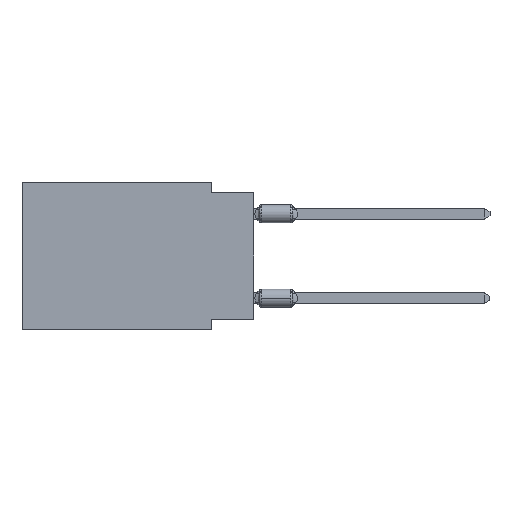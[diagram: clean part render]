
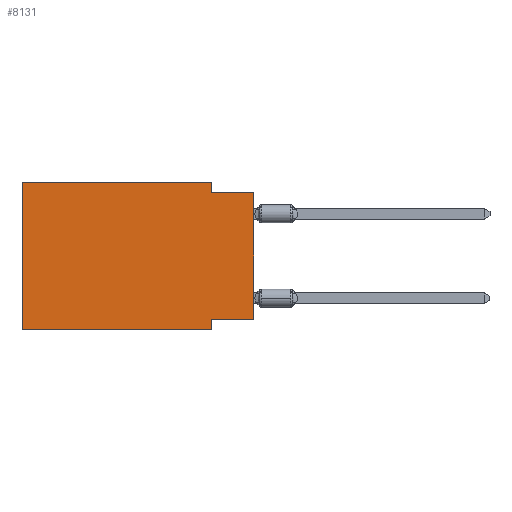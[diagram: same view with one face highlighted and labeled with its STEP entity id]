
A CAD part, left-side view. The second image highlights one B-rep face of the part: STEP entity #8131.
In plain terms, the highlighted planar face has unit normal (-1, 0, 0).
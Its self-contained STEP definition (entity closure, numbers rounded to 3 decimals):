
#757 = LINE ( 'NONE', #5608, #9518 ) ;
#918 = CARTESIAN_POINT ( 'NONE',  ( 0., 2.54, 0. ) ) ;
#1144 = CARTESIAN_POINT ( 'NONE',  ( 0., 0., -8.255 ) ) ;
#1359 = FACE_OUTER_BOUND ( 'NONE', #2654, .T. ) ;
#1428 = ORIENTED_EDGE ( 'NONE', *, *, #14128, .F. ) ;
#1642 = VERTEX_POINT ( 'NONE', #2479 ) ;
#1798 = CARTESIAN_POINT ( 'NONE',  ( 0., 2.54, 0. ) ) ;
#2180 = DIRECTION ( 'NONE',  ( 0., -1., 0. ) ) ;
#2479 = CARTESIAN_POINT ( 'NONE',  ( 0., 0., -8.255 ) ) ;
#2654 = EDGE_LOOP ( 'NONE', ( #10123, #14955, #10845, #11488, #1428, #11144, #3046, #14846 ) ) ;
#2805 = VERTEX_POINT ( 'NONE', #5800 ) ;
#3046 = ORIENTED_EDGE ( 'NONE', *, *, #6299, .F. ) ;
#4179 = DIRECTION ( 'NONE',  ( 0., 0., -1. ) ) ;
#4244 = VERTEX_POINT ( 'NONE', #5640 ) ;
#4555 = VERTEX_POINT ( 'NONE', #7541 ) ;
#4774 = LINE ( 'NONE', #12886, #14269 ) ;
#5047 = LINE ( 'NONE', #8569, #7415 ) ;
#5528 = DIRECTION ( 'NONE',  ( 0., 0., -1. ) ) ;
#5608 = CARTESIAN_POINT ( 'NONE',  ( 0., 0., -0.635 ) ) ;
#5640 = CARTESIAN_POINT ( 'NONE',  ( 0., 2.54, -8.255 ) ) ;
#5800 = CARTESIAN_POINT ( 'NONE',  ( 0., 2.54, -0.635 ) ) ;
#6046 = CARTESIAN_POINT ( 'NONE',  ( 0., 13.97, 0. ) ) ;
#6086 = DIRECTION ( 'NONE',  ( 0., 0., 1. ) ) ;
#6299 = EDGE_CURVE ( 'NONE', #4244, #14451, #6594, .T. ) ;
#6594 = LINE ( 'NONE', #10121, #6756 ) ;
#6756 = VECTOR ( 'NONE', #5528, 1000. ) ;
#7365 = VERTEX_POINT ( 'NONE', #7749 ) ;
#7415 = VECTOR ( 'NONE', #12149, 1000. ) ;
#7452 = CARTESIAN_POINT ( 'NONE',  ( 0., 13.97, -8.89 ) ) ;
#7541 = CARTESIAN_POINT ( 'NONE',  ( 0., 13.97, -8.89 ) ) ;
#7600 = LINE ( 'NONE', #7452, #10975 ) ;
#7635 = DIRECTION ( 'NONE',  ( 0., 0., -1. ) ) ;
#7644 = EDGE_CURVE ( 'NONE', #1642, #4244, #13018, .T. ) ;
#7749 = CARTESIAN_POINT ( 'NONE',  ( 0., 0., -0.635 ) ) ;
#8131 = ADVANCED_FACE ( 'NONE', ( #1359 ), #10775, .F. ) ;
#8351 = DIRECTION ( 'NONE',  ( 0., 1., 0. ) ) ;
#8569 = CARTESIAN_POINT ( 'NONE',  ( 0., 13.97, 0. ) ) ;
#8649 = VECTOR ( 'NONE', #2180, 1000. ) ;
#9145 = DIRECTION ( 'NONE',  ( 0., -1., 0. ) ) ;
#9284 = EDGE_CURVE ( 'NONE', #4555, #14451, #7600, .T. ) ;
#9467 = EDGE_CURVE ( 'NONE', #2805, #7365, #757, .T. ) ;
#9518 = VECTOR ( 'NONE', #9145, 1000. ) ;
#9781 = VECTOR ( 'NONE', #4179, 1000. ) ;
#10121 = CARTESIAN_POINT ( 'NONE',  ( 0., 2.54, -8.89 ) ) ;
#10123 = ORIENTED_EDGE ( 'NONE', *, *, #13131, .T. ) ;
#10190 = EDGE_CURVE ( 'NONE', #10727, #2805, #12273, .T. ) ;
#10671 = VERTEX_POINT ( 'NONE', #13940 ) ;
#10700 = DIRECTION ( 'NONE',  ( 1., 0., 0. ) ) ;
#10727 = VERTEX_POINT ( 'NONE', #918 ) ;
#10775 = PLANE ( 'NONE',  #11704 ) ;
#10845 = ORIENTED_EDGE ( 'NONE', *, *, #10190, .F. ) ;
#10975 = VECTOR ( 'NONE', #14346, 1000. ) ;
#11144 = ORIENTED_EDGE ( 'NONE', *, *, #9284, .T. ) ;
#11488 = ORIENTED_EDGE ( 'NONE', *, *, #12997, .F. ) ;
#11704 = AXIS2_PLACEMENT_3D ( 'NONE', #6046, #10700, #7635 ) ;
#12149 = DIRECTION ( 'NONE',  ( 0., 0., 1. ) ) ;
#12156 = VECTOR ( 'NONE', #8351, 1000. ) ;
#12273 = LINE ( 'NONE', #1798, #9781 ) ;
#12504 = CARTESIAN_POINT ( 'NONE',  ( 0., 13.97, 0. ) ) ;
#12886 = CARTESIAN_POINT ( 'NONE',  ( 0., 0., 0. ) ) ;
#12997 = EDGE_CURVE ( 'NONE', #10671, #10727, #13733, .T. ) ;
#13018 = LINE ( 'NONE', #1144, #12156 ) ;
#13131 = EDGE_CURVE ( 'NONE', #1642, #7365, #4774, .T. ) ;
#13191 = CARTESIAN_POINT ( 'NONE',  ( 0., 2.54, -8.89 ) ) ;
#13733 = LINE ( 'NONE', #12504, #8649 ) ;
#13940 = CARTESIAN_POINT ( 'NONE',  ( 0., 13.97, 0. ) ) ;
#14128 = EDGE_CURVE ( 'NONE', #4555, #10671, #5047, .T. ) ;
#14269 = VECTOR ( 'NONE', #6086, 1000. ) ;
#14346 = DIRECTION ( 'NONE',  ( 0., -1., 0. ) ) ;
#14451 = VERTEX_POINT ( 'NONE', #13191 ) ;
#14846 = ORIENTED_EDGE ( 'NONE', *, *, #7644, .F. ) ;
#14955 = ORIENTED_EDGE ( 'NONE', *, *, #9467, .F. ) ;
